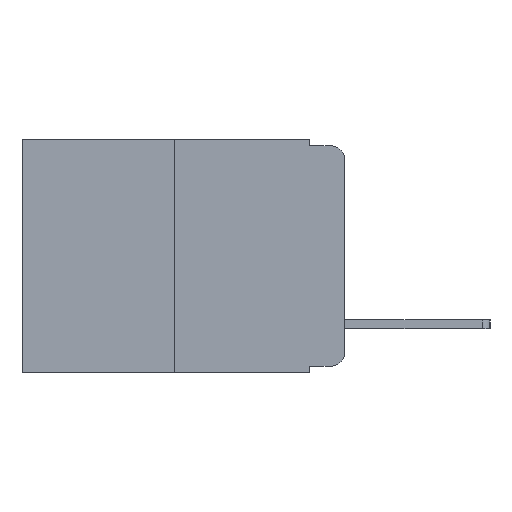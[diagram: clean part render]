
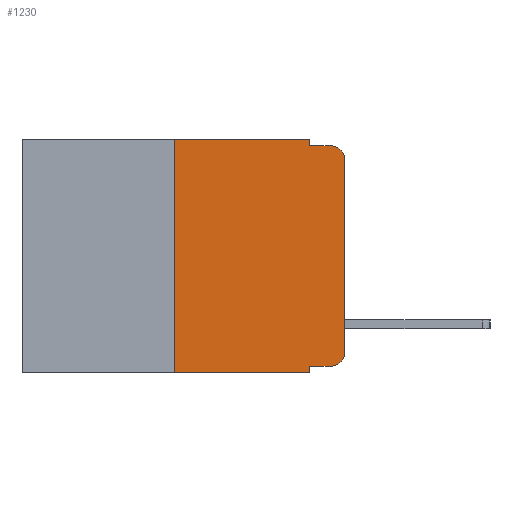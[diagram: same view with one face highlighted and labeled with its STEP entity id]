
A CAD part, left-side view. The second image highlights one B-rep face of the part: STEP entity #1230.
In plain terms, the highlighted planar face has unit normal (-1, 0, 0).
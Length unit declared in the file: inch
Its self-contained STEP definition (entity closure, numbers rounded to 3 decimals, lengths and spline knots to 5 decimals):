
#120 = VECTOR ( 'NONE', #10823, 39.37008 ) ;
#159 = CARTESIAN_POINT ( 'NONE',  ( 0., 0.25, -0.343 ) ) ;
#217 = DIRECTION ( 'NONE',  ( 0., 0., 1. ) ) ;
#502 = CARTESIAN_POINT ( 'NONE',  ( 0., 0.473, -0.343 ) ) ;
#872 = EDGE_CURVE ( 'NONE', #3444, #3212, #5270, .T. ) ;
#908 = VERTEX_POINT ( 'NONE', #6409 ) ;
#936 = VERTEX_POINT ( 'NONE', #8212 ) ;
#1039 = CARTESIAN_POINT ( 'NONE',  ( 0., 0.25, 0. ) ) ;
#1167 = LINE ( 'NONE', #2301, #10120 ) ;
#1230 = ADVANCED_FACE ( 'NONE', ( #3992 ), #7555, .F. ) ;
#1354 = ORIENTED_EDGE ( 'NONE', *, *, #1644, .F. ) ;
#1438 = CARTESIAN_POINT ( 'NONE',  ( 0., 0.051, -0.333 ) ) ;
#1495 = LINE ( 'NONE', #1039, #3995 ) ;
#1644 = EDGE_CURVE ( 'NONE', #5737, #3444, #1495, .T. ) ;
#1806 = EDGE_CURVE ( 'NONE', #908, #6378, #9160, .T. ) ;
#2055 = LINE ( 'NONE', #502, #10849 ) ;
#2073 = CARTESIAN_POINT ( 'NONE',  ( 0., 0.051, -0.01 ) ) ;
#2301 = CARTESIAN_POINT ( 'NONE',  ( 0., 0., 0. ) ) ;
#2559 = VECTOR ( 'NONE', #6569, 39.37008 ) ;
#2579 = ORIENTED_EDGE ( 'NONE', *, *, #1806, .T. ) ;
#2595 = DIRECTION ( 'NONE',  ( 0., -1., 0. ) ) ;
#2702 = CARTESIAN_POINT ( 'NONE',  ( 0., 0.051, -0.343 ) ) ;
#2733 = LINE ( 'NONE', #5051, #120 ) ;
#2734 = ORIENTED_EDGE ( 'NONE', *, *, #4188, .T. ) ;
#2739 = ORIENTED_EDGE ( 'NONE', *, *, #9267, .T. ) ;
#2751 = ORIENTED_EDGE ( 'NONE', *, *, #3284, .T. ) ;
#3212 = VERTEX_POINT ( 'NONE', #9278 ) ;
#3284 = EDGE_CURVE ( 'NONE', #936, #908, #1167, .T. ) ;
#3444 = VERTEX_POINT ( 'NONE', #11017 ) ;
#3509 = VECTOR ( 'NONE', #3569, 39.37008 ) ;
#3512 = VERTEX_POINT ( 'NONE', #2702 ) ;
#3521 = AXIS2_PLACEMENT_3D ( 'NONE', #8353, #4143, #8255 ) ;
#3569 = DIRECTION ( 'NONE',  ( 0., 0., -1. ) ) ;
#3992 = FACE_OUTER_BOUND ( 'NONE', #10572, .T. ) ;
#3995 = VECTOR ( 'NONE', #10972, 39.37008 ) ;
#4001 = CIRCLE ( 'NONE', #10029, 0.02 ) ;
#4049 = EDGE_CURVE ( 'NONE', #9849, #3512, #8135, .T. ) ;
#4143 = DIRECTION ( 'NONE',  ( -1., 0., 0. ) ) ;
#4188 = EDGE_CURVE ( 'NONE', #9849, #8295, #11095, .T. ) ;
#4537 = CARTESIAN_POINT ( 'NONE',  ( 0., 0.02, -0.313 ) ) ;
#4651 = ORIENTED_EDGE ( 'NONE', *, *, #10921, .T. ) ;
#4745 = ORIENTED_EDGE ( 'NONE', *, *, #872, .F. ) ;
#5051 = CARTESIAN_POINT ( 'NONE',  ( 0., 0.051, 0. ) ) ;
#5086 = ORIENTED_EDGE ( 'NONE', *, *, #5714, .F. ) ;
#5270 = LINE ( 'NONE', #6603, #2559 ) ;
#5454 = DIRECTION ( 'NONE',  ( 0., 0., -1. ) ) ;
#5714 = EDGE_CURVE ( 'NONE', #10614, #6378, #10080, .T. ) ;
#5737 = VERTEX_POINT ( 'NONE', #159 ) ;
#6011 = ORIENTED_EDGE ( 'NONE', *, *, #7178, .F. ) ;
#6378 = VERTEX_POINT ( 'NONE', #8278 ) ;
#6409 = CARTESIAN_POINT ( 'NONE',  ( 0., 0., -0.03 ) ) ;
#6569 = DIRECTION ( 'NONE',  ( 0., -1., 0. ) ) ;
#6603 = CARTESIAN_POINT ( 'NONE',  ( 0., 0.473, 0. ) ) ;
#7178 = EDGE_CURVE ( 'NONE', #3212, #10614, #2733, .T. ) ;
#7210 = CARTESIAN_POINT ( 'NONE',  ( 0., 0.473, 0. ) ) ;
#7378 = CARTESIAN_POINT ( 'NONE',  ( 0., 0.051, -0.01 ) ) ;
#7555 = PLANE ( 'NONE',  #10682 ) ;
#8042 = ORIENTED_EDGE ( 'NONE', *, *, #4049, .F. ) ;
#8135 = LINE ( 'NONE', #10296, #3509 ) ;
#8212 = CARTESIAN_POINT ( 'NONE',  ( 0., 0., -0.313 ) ) ;
#8255 = DIRECTION ( 'NONE',  ( 0., 0., -1. ) ) ;
#8278 = CARTESIAN_POINT ( 'NONE',  ( 0., 0.02, -0.01 ) ) ;
#8295 = VERTEX_POINT ( 'NONE', #9664 ) ;
#8353 = CARTESIAN_POINT ( 'NONE',  ( 0., 0.02, -0.03 ) ) ;
#8970 = VECTOR ( 'NONE', #9030, 39.37008 ) ;
#8995 = VECTOR ( 'NONE', #9622, 39.37008 ) ;
#9030 = DIRECTION ( 'NONE',  ( 0., -1., 0. ) ) ;
#9160 = CIRCLE ( 'NONE', #3521, 0.02 ) ;
#9267 = EDGE_CURVE ( 'NONE', #8295, #936, #4001, .T. ) ;
#9278 = CARTESIAN_POINT ( 'NONE',  ( 0., 0.051, 0. ) ) ;
#9526 = CARTESIAN_POINT ( 'NONE',  ( 0., 0.051, -0.333 ) ) ;
#9622 = DIRECTION ( 'NONE',  ( 0., -1., 0. ) ) ;
#9664 = CARTESIAN_POINT ( 'NONE',  ( 0., 0.02, -0.333 ) ) ;
#9849 = VERTEX_POINT ( 'NONE', #9526 ) ;
#10029 = AXIS2_PLACEMENT_3D ( 'NONE', #4537, #10339, #5454 ) ;
#10080 = LINE ( 'NONE', #2073, #8970 ) ;
#10120 = VECTOR ( 'NONE', #217, 39.37008 ) ;
#10296 = CARTESIAN_POINT ( 'NONE',  ( 0., 0.051, 0. ) ) ;
#10339 = DIRECTION ( 'NONE',  ( -1., 0., 0. ) ) ;
#10572 = EDGE_LOOP ( 'NONE', ( #2751, #2579, #5086, #6011, #4745, #1354, #4651, #8042, #2734, #2739 ) ) ;
#10614 = VERTEX_POINT ( 'NONE', #7378 ) ;
#10682 = AXIS2_PLACEMENT_3D ( 'NONE', #7210, #11055, #11112 ) ;
#10823 = DIRECTION ( 'NONE',  ( 0., 0., -1. ) ) ;
#10849 = VECTOR ( 'NONE', #2595, 39.37008 ) ;
#10921 = EDGE_CURVE ( 'NONE', #5737, #3512, #2055, .T. ) ;
#10972 = DIRECTION ( 'NONE',  ( 0., 0., 1. ) ) ;
#11017 = CARTESIAN_POINT ( 'NONE',  ( 0., 0.25, 0. ) ) ;
#11055 = DIRECTION ( 'NONE',  ( 1., 0., 0. ) ) ;
#11095 = LINE ( 'NONE', #1438, #8995 ) ;
#11112 = DIRECTION ( 'NONE',  ( 0., 0., -1. ) ) ;
